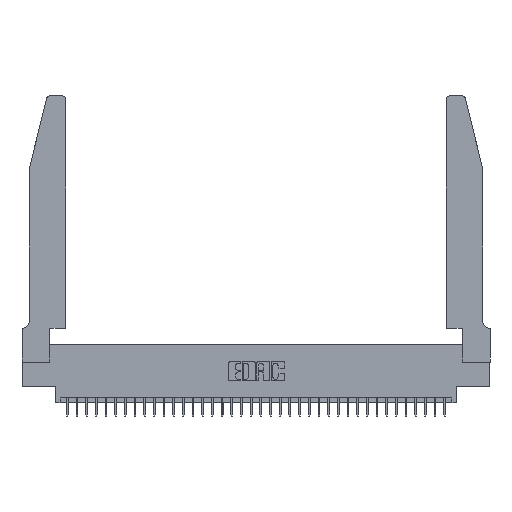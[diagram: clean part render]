
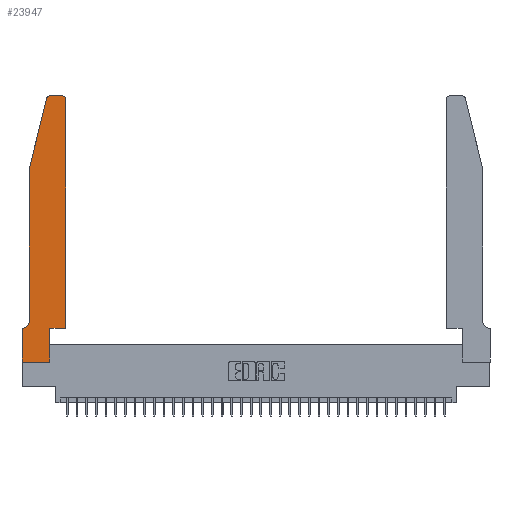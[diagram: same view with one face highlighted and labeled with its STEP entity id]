
A CAD part, top view. The second image highlights one B-rep face of the part: STEP entity #23947.
In plain terms, the highlighted planar face has unit normal (0, 0, 1).
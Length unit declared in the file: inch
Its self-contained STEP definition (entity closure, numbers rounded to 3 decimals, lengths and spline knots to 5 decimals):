
#261 = EDGE_LOOP ( 'NONE', ( #13718, #4347, #28696, #8415, #6073, #29119, #5241, #6545, #3281, #7678, #6725, #26784 ) ) ;
#520 = VERTEX_POINT ( 'NONE', #24809 ) ;
#790 = CARTESIAN_POINT ( 'NONE',  ( 0.2865, 0.35, 0.37 ) ) ;
#830 = CARTESIAN_POINT ( 'NONE',  ( 0.0755, 2., 0.37 ) ) ;
#960 = EDGE_CURVE ( 'NONE', #13230, #23854, #34339, .T. ) ;
#1380 = DIRECTION ( 'NONE',  ( 0., 0., -1. ) ) ;
#1677 = EDGE_CURVE ( 'NONE', #27232, #13230, #19599, .T. ) ;
#1774 = CARTESIAN_POINT ( 'NONE',  ( 0.284, 2.72, 0.37 ) ) ;
#2122 = DIRECTION ( 'NONE',  ( 0., -1., 0. ) ) ;
#2492 = CIRCLE ( 'NONE', #22037, 0.07 ) ;
#3281 = ORIENTED_EDGE ( 'NONE', *, *, #1677, .T. ) ;
#3505 = VECTOR ( 'NONE', #14333, 39.37008 ) ;
#3561 = VECTOR ( 'NONE', #7561, 39.37008 ) ;
#4298 = CARTESIAN_POINT ( 'NONE',  ( 0.2865, 0., 0.37 ) ) ;
#4347 = ORIENTED_EDGE ( 'NONE', *, *, #33128, .T. ) ;
#4364 = EDGE_CURVE ( 'NONE', #9437, #520, #24113, .T. ) ;
#5241 = ORIENTED_EDGE ( 'NONE', *, *, #21522, .T. ) ;
#5330 = EDGE_CURVE ( 'NONE', #24804, #22619, #20051, .T. ) ;
#5840 = EDGE_CURVE ( 'NONE', #23854, #9709, #16846, .T. ) ;
#6073 = ORIENTED_EDGE ( 'NONE', *, *, #11362, .T. ) ;
#6318 = CARTESIAN_POINT ( 'NONE',  ( 0., 0., 0.37 ) ) ;
#6545 = ORIENTED_EDGE ( 'NONE', *, *, #20209, .T. ) ;
#6725 = ORIENTED_EDGE ( 'NONE', *, *, #5840, .T. ) ;
#7561 = DIRECTION ( 'NONE',  ( 0., 1., 0. ) ) ;
#7678 = ORIENTED_EDGE ( 'NONE', *, *, #960, .T. ) ;
#8177 = DIRECTION ( 'NONE',  ( -0.239, -0.971, 0. ) ) ;
#8415 = ORIENTED_EDGE ( 'NONE', *, *, #12884, .T. ) ;
#8940 = DIRECTION ( 'NONE',  ( 1., 0., 0. ) ) ;
#9129 = LINE ( 'NONE', #28407, #3505 ) ;
#9437 = VERTEX_POINT ( 'NONE', #11684 ) ;
#9709 = VERTEX_POINT ( 'NONE', #16069 ) ;
#9918 = DIRECTION ( 'NONE',  ( 0., 0., 1. ) ) ;
#10822 = LINE ( 'NONE', #22115, #14402 ) ;
#10977 = CARTESIAN_POINT ( 'NONE',  ( 0.0755, 2., 0.37 ) ) ;
#11117 = DIRECTION ( 'NONE',  ( 0., 1., 0. ) ) ;
#11201 = CARTESIAN_POINT ( 'NONE',  ( 0., 0., 0.37 ) ) ;
#11246 = AXIS2_PLACEMENT_3D ( 'NONE', #26162, #29490, #12459 ) ;
#11362 = EDGE_CURVE ( 'NONE', #31782, #9437, #2492, .T. ) ;
#11684 = CARTESIAN_POINT ( 'NONE',  ( 0.0055, 0.35, 0.37 ) ) ;
#11750 = CARTESIAN_POINT ( 'NONE',  ( 0.4505, 0.35, 0.37 ) ) ;
#12444 = VECTOR ( 'NONE', #14883, 39.37008 ) ;
#12459 = DIRECTION ( 'NONE',  ( 1., 0., 0. ) ) ;
#12884 = EDGE_CURVE ( 'NONE', #22619, #31782, #24400, .T. ) ;
#13087 = CARTESIAN_POINT ( 'NONE',  ( 0.0755, 0.42, 0.37 ) ) ;
#13230 = VERTEX_POINT ( 'NONE', #790 ) ;
#13718 = ORIENTED_EDGE ( 'NONE', *, *, #24133, .T. ) ;
#14333 = DIRECTION ( 'NONE',  ( 0., -1., 0. ) ) ;
#14402 = VECTOR ( 'NONE', #28785, 39.37008 ) ;
#14883 = DIRECTION ( 'NONE',  ( 1., 0., 0. ) ) ;
#15923 = VECTOR ( 'NONE', #32615, 39.37008 ) ;
#16069 = CARTESIAN_POINT ( 'NONE',  ( 0.4505, 2.72, 0.37 ) ) ;
#16524 = VERTEX_POINT ( 'NONE', #21995 ) ;
#16846 = LINE ( 'NONE', #25209, #35876 ) ;
#16977 = VERTEX_POINT ( 'NONE', #31250 ) ;
#17278 = LINE ( 'NONE', #6318, #17680 ) ;
#17680 = VECTOR ( 'NONE', #8940, 39.37008 ) ;
#18818 = AXIS2_PLACEMENT_3D ( 'NONE', #1774, #24433, #35721 ) ;
#19598 = CARTESIAN_POINT ( 'NONE',  ( 0.4505, 0.35, 0.37 ) ) ;
#19599 = LINE ( 'NONE', #30555, #3561 ) ;
#20051 = LINE ( 'NONE', #10977, #35610 ) ;
#20209 = EDGE_CURVE ( 'NONE', #24168, #27232, #17278, .T. ) ;
#20698 = CARTESIAN_POINT ( 'NONE',  ( 0.0055, 0.42, 0.37 ) ) ;
#20873 = DIRECTION ( 'NONE',  ( -1., 0., 0. ) ) ;
#21221 = DIRECTION ( 'NONE',  ( 1., 0., 0. ) ) ;
#21522 = EDGE_CURVE ( 'NONE', #520, #24168, #9129, .T. ) ;
#21995 = CARTESIAN_POINT ( 'NONE',  ( 0.4205, 2.75, 0.37 ) ) ;
#22037 = AXIS2_PLACEMENT_3D ( 'NONE', #20698, #1380, #20873 ) ;
#22115 = CARTESIAN_POINT ( 'NONE',  ( 0.2605, 2.75, 0.37 ) ) ;
#22619 = VERTEX_POINT ( 'NONE', #830 ) ;
#23854 = VERTEX_POINT ( 'NONE', #19598 ) ;
#23947 = ADVANCED_FACE ( 'NONE', ( #26783 ), #35297, .T. ) ;
#24113 = LINE ( 'NONE', #30384, #15923 ) ;
#24133 = EDGE_CURVE ( 'NONE', #16524, #16977, #10822, .T. ) ;
#24168 = VERTEX_POINT ( 'NONE', #11201 ) ;
#24400 = LINE ( 'NONE', #33281, #34559 ) ;
#24433 = DIRECTION ( 'NONE',  ( 0., 0., 1. ) ) ;
#24804 = VERTEX_POINT ( 'NONE', #34470 ) ;
#24809 = CARTESIAN_POINT ( 'NONE',  ( 0., 0.35, 0.37 ) ) ;
#25209 = CARTESIAN_POINT ( 'NONE',  ( 0.4505, 0.35, 0.37 ) ) ;
#26162 = CARTESIAN_POINT ( 'NONE',  ( 0.4205, 2.72, 0.37 ) ) ;
#26226 = CARTESIAN_POINT ( 'NONE',  ( 0., 0.35, 0.37 ) ) ;
#26783 = FACE_OUTER_BOUND ( 'NONE', #261, .T. ) ;
#26784 = ORIENTED_EDGE ( 'NONE', *, *, #36131, .T. ) ;
#27232 = VERTEX_POINT ( 'NONE', #4298 ) ;
#28407 = CARTESIAN_POINT ( 'NONE',  ( 0., 0., 0.37 ) ) ;
#28606 = AXIS2_PLACEMENT_3D ( 'NONE', #26226, #9918, #21221 ) ;
#28696 = ORIENTED_EDGE ( 'NONE', *, *, #5330, .T. ) ;
#28785 = DIRECTION ( 'NONE',  ( -1., 0., 0. ) ) ;
#29119 = ORIENTED_EDGE ( 'NONE', *, *, #4364, .T. ) ;
#29490 = DIRECTION ( 'NONE',  ( 0., 0., 1. ) ) ;
#30384 = CARTESIAN_POINT ( 'NONE',  ( 0.0755, 0.35, 0.37 ) ) ;
#30555 = CARTESIAN_POINT ( 'NONE',  ( 0.2865, 0.35, 0.37 ) ) ;
#31250 = CARTESIAN_POINT ( 'NONE',  ( 0.284, 2.75, 0.37 ) ) ;
#31782 = VERTEX_POINT ( 'NONE', #13087 ) ;
#32564 = CIRCLE ( 'NONE', #11246, 0.03 ) ;
#32615 = DIRECTION ( 'NONE',  ( -1., 0., 0. ) ) ;
#33128 = EDGE_CURVE ( 'NONE', #16977, #24804, #35364, .T. ) ;
#33281 = CARTESIAN_POINT ( 'NONE',  ( 0.0755, 2., 0.37 ) ) ;
#34339 = LINE ( 'NONE', #11750, #12444 ) ;
#34470 = CARTESIAN_POINT ( 'NONE',  ( 0.25487, 2.72718, 0.37 ) ) ;
#34559 = VECTOR ( 'NONE', #2122, 39.37008 ) ;
#35297 = PLANE ( 'NONE',  #28606 ) ;
#35364 = CIRCLE ( 'NONE', #18818, 0.03 ) ;
#35610 = VECTOR ( 'NONE', #8177, 39.37008 ) ;
#35721 = DIRECTION ( 'NONE',  ( 1., 0., 0. ) ) ;
#35876 = VECTOR ( 'NONE', #11117, 39.37008 ) ;
#36131 = EDGE_CURVE ( 'NONE', #9709, #16524, #32564, .T. ) ;
